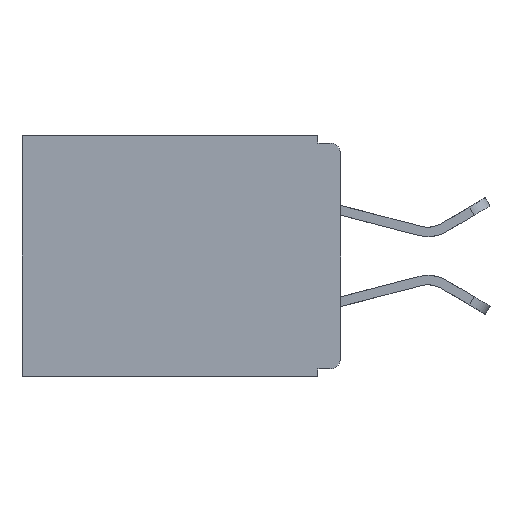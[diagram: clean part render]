
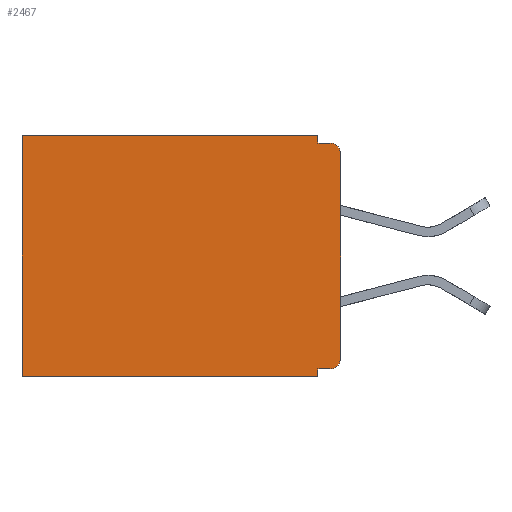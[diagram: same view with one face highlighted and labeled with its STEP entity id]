
A CAD part, left-side view. The second image highlights one B-rep face of the part: STEP entity #2467.
In plain terms, the highlighted planar face has unit normal (-1, 0, 0).
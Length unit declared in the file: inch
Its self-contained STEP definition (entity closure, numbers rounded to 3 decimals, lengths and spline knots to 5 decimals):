
#307 = ORIENTED_EDGE ( 'NONE', *, *, #10265, .T. ) ;
#337 = VERTEX_POINT ( 'NONE', #2153 ) ;
#428 = DIRECTION ( 'NONE',  ( 0., -1., 0. ) ) ;
#593 = DIRECTION ( 'NONE',  ( 0., 0., -1. ) ) ;
#679 = VECTOR ( 'NONE', #5092, 39.37008 ) ;
#1209 = EDGE_CURVE ( 'NONE', #337, #2775, #1356, .T. ) ;
#1246 = ORIENTED_EDGE ( 'NONE', *, *, #2423, .F. ) ;
#1305 = CARTESIAN_POINT ( 'NONE',  ( 0.3, 0.031, -0.33 ) ) ;
#1356 = CIRCLE ( 'NONE', #6456, 0.015 ) ;
#1745 = VECTOR ( 'NONE', #6778, 39.37008 ) ;
#1762 = LINE ( 'NONE', #5046, #679 ) ;
#1955 = EDGE_CURVE ( 'NONE', #10924, #3240, #10906, .T. ) ;
#2152 = VECTOR ( 'NONE', #428, 39.37008 ) ;
#2153 = CARTESIAN_POINT ( 'NONE',  ( 0.3, 0.015, -0.32 ) ) ;
#2294 = ORIENTED_EDGE ( 'NONE', *, *, #8257, .T. ) ;
#2347 = CARTESIAN_POINT ( 'NONE',  ( 0.3, 0.015, -0.025 ) ) ;
#2422 = CARTESIAN_POINT ( 'NONE',  ( 0.3, 0., -0.33 ) ) ;
#2423 = EDGE_CURVE ( 'NONE', #10149, #2775, #5914, .T. ) ;
#2467 = ADVANCED_FACE ( 'NONE', ( #2777 ), #7742, .F. ) ;
#2648 = ORIENTED_EDGE ( 'NONE', *, *, #1955, .F. ) ;
#2775 = VERTEX_POINT ( 'NONE', #4026 ) ;
#2777 = FACE_OUTER_BOUND ( 'NONE', #5708, .T. ) ;
#3240 = VERTEX_POINT ( 'NONE', #1305 ) ;
#3326 = DIRECTION ( 'NONE',  ( 0., 1., 0. ) ) ;
#3355 = CARTESIAN_POINT ( 'NONE',  ( 0.3, 0., -0.33 ) ) ;
#3580 = CARTESIAN_POINT ( 'NONE',  ( 0.3, 0.437, -0.33 ) ) ;
#3799 = ORIENTED_EDGE ( 'NONE', *, *, #4399, .F. ) ;
#3900 = CARTESIAN_POINT ( 'NONE',  ( 0.3, 0.031, -0.33 ) ) ;
#4026 = CARTESIAN_POINT ( 'NONE',  ( 0.3, 0., -0.305 ) ) ;
#4097 = DIRECTION ( 'NONE',  ( -1., 0., 0. ) ) ;
#4111 = ORIENTED_EDGE ( 'NONE', *, *, #10117, .F. ) ;
#4285 = ORIENTED_EDGE ( 'NONE', *, *, #10771, .F. ) ;
#4399 = EDGE_CURVE ( 'NONE', #10074, #8403, #9014, .T. ) ;
#4443 = LINE ( 'NONE', #8318, #5263 ) ;
#4559 = CARTESIAN_POINT ( 'NONE',  ( 0.3, 0.031, -0.32 ) ) ;
#4711 = DIRECTION ( 'NONE',  ( -1., 0., 0. ) ) ;
#4970 = DIRECTION ( 'NONE',  ( 0., 0., -1. ) ) ;
#5041 = CIRCLE ( 'NONE', #9819, 0.015 ) ;
#5046 = CARTESIAN_POINT ( 'NONE',  ( 0.3, 0., 0. ) ) ;
#5092 = DIRECTION ( 'NONE',  ( 0., 1., 0. ) ) ;
#5156 = CARTESIAN_POINT ( 'NONE',  ( 0.3, 0.031, 0. ) ) ;
#5263 = VECTOR ( 'NONE', #593, 39.37008 ) ;
#5286 = CARTESIAN_POINT ( 'NONE',  ( 0.3, 0.031, -0.01 ) ) ;
#5347 = LINE ( 'NONE', #9289, #7210 ) ;
#5607 = CARTESIAN_POINT ( 'NONE',  ( 0.3, 0.437, 0. ) ) ;
#5657 = LINE ( 'NONE', #3355, #1745 ) ;
#5662 = VECTOR ( 'NONE', #9788, 39.37008 ) ;
#5708 = EDGE_LOOP ( 'NONE', ( #1246, #2294, #3799, #4111, #307, #8139, #4285, #2648, #10005, #9192 ) ) ;
#5750 = CARTESIAN_POINT ( 'NONE',  ( 0.3, 0., -0.33 ) ) ;
#5870 = DIRECTION ( 'NONE',  ( 0., 0., -1. ) ) ;
#5876 = VERTEX_POINT ( 'NONE', #5607 ) ;
#5914 = LINE ( 'NONE', #5750, #11036 ) ;
#6032 = AXIS2_PLACEMENT_3D ( 'NONE', #2422, #8610, #7710 ) ;
#6356 = EDGE_CURVE ( 'NONE', #5876, #8474, #5347, .T. ) ;
#6456 = AXIS2_PLACEMENT_3D ( 'NONE', #8165, #4711, #10739 ) ;
#6710 = CARTESIAN_POINT ( 'NONE',  ( 0.3, 0., -0.32 ) ) ;
#6778 = DIRECTION ( 'NONE',  ( 0., 1., 0. ) ) ;
#6937 = CARTESIAN_POINT ( 'NONE',  ( 0.3, 0.015, -0.01 ) ) ;
#7210 = VECTOR ( 'NONE', #5870, 39.37008 ) ;
#7411 = CARTESIAN_POINT ( 'NONE',  ( 0.3, 0., -0.01 ) ) ;
#7710 = DIRECTION ( 'NONE',  ( 0., 0., -1. ) ) ;
#7742 = PLANE ( 'NONE',  #6032 ) ;
#8139 = ORIENTED_EDGE ( 'NONE', *, *, #6356, .T. ) ;
#8165 = CARTESIAN_POINT ( 'NONE',  ( 0.3, 0.015, -0.305 ) ) ;
#8257 = EDGE_CURVE ( 'NONE', #10149, #8403, #5041, .T. ) ;
#8318 = CARTESIAN_POINT ( 'NONE',  ( 0.3, 0.031, 0. ) ) ;
#8403 = VERTEX_POINT ( 'NONE', #6937 ) ;
#8412 = VERTEX_POINT ( 'NONE', #5156 ) ;
#8422 = DIRECTION ( 'NONE',  ( 0., 0., -1. ) ) ;
#8474 = VERTEX_POINT ( 'NONE', #3580 ) ;
#8610 = DIRECTION ( 'NONE',  ( 1., 0., 0. ) ) ;
#9014 = LINE ( 'NONE', #7411, #2152 ) ;
#9167 = VECTOR ( 'NONE', #3326, 39.37008 ) ;
#9192 = ORIENTED_EDGE ( 'NONE', *, *, #1209, .T. ) ;
#9289 = CARTESIAN_POINT ( 'NONE',  ( 0.3, 0.437, -0.33 ) ) ;
#9450 = LINE ( 'NONE', #6710, #9167 ) ;
#9737 = EDGE_CURVE ( 'NONE', #337, #10924, #9450, .T. ) ;
#9788 = DIRECTION ( 'NONE',  ( 0., 0., -1. ) ) ;
#9819 = AXIS2_PLACEMENT_3D ( 'NONE', #2347, #4097, #4970 ) ;
#10005 = ORIENTED_EDGE ( 'NONE', *, *, #9737, .F. ) ;
#10025 = CARTESIAN_POINT ( 'NONE',  ( 0.3, 0., -0.025 ) ) ;
#10074 = VERTEX_POINT ( 'NONE', #5286 ) ;
#10117 = EDGE_CURVE ( 'NONE', #8412, #10074, #4443, .T. ) ;
#10149 = VERTEX_POINT ( 'NONE', #10025 ) ;
#10265 = EDGE_CURVE ( 'NONE', #8412, #5876, #1762, .T. ) ;
#10739 = DIRECTION ( 'NONE',  ( 0., 0., -1. ) ) ;
#10771 = EDGE_CURVE ( 'NONE', #3240, #8474, #5657, .T. ) ;
#10906 = LINE ( 'NONE', #3900, #5662 ) ;
#10924 = VERTEX_POINT ( 'NONE', #4559 ) ;
#11036 = VECTOR ( 'NONE', #8422, 39.37008 ) ;
